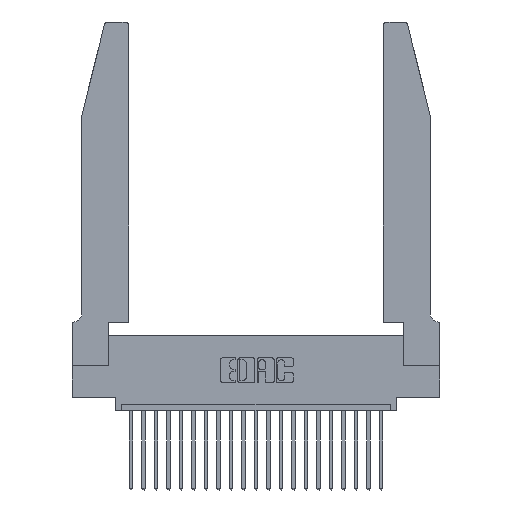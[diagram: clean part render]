
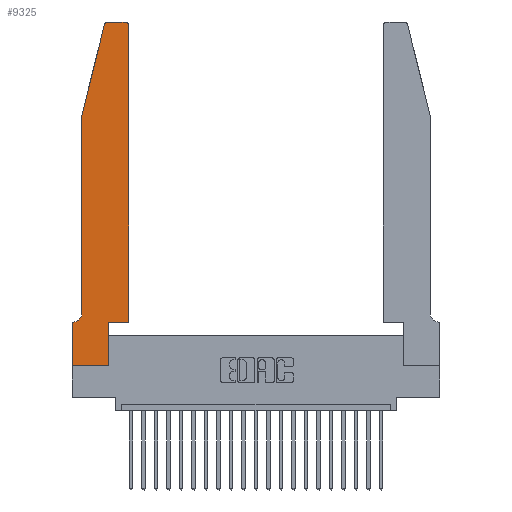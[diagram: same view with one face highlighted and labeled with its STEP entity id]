
A CAD part, top view. The second image highlights one B-rep face of the part: STEP entity #9325.
In plain terms, the highlighted planar face has unit normal (0, 0, 1).
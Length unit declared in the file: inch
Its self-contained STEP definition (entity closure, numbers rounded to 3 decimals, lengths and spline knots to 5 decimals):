
#267 = CARTESIAN_POINT ( 'NONE',  ( 0.0755, 2., 0.37 ) ) ;
#661 = VECTOR ( 'NONE', #10644, 39.37008 ) ;
#750 = VECTOR ( 'NONE', #2296, 39.37008 ) ;
#885 = ORIENTED_EDGE ( 'NONE', *, *, #1865, .T. ) ;
#1027 = CARTESIAN_POINT ( 'NONE',  ( 0.0755, 2., 0.37 ) ) ;
#1036 = CARTESIAN_POINT ( 'NONE',  ( 0., 0., 0.37 ) ) ;
#1344 = LINE ( 'NONE', #19216, #16714 ) ;
#1485 = FACE_OUTER_BOUND ( 'NONE', #23130, .T. ) ;
#1508 = CARTESIAN_POINT ( 'NONE',  ( 0.0055, 0.35, 0.37 ) ) ;
#1568 = EDGE_CURVE ( 'NONE', #22589, #5425, #1344, .T. ) ;
#1865 = EDGE_CURVE ( 'NONE', #16413, #19247, #22656, .T. ) ;
#2060 = ORIENTED_EDGE ( 'NONE', *, *, #14155, .T. ) ;
#2296 = DIRECTION ( 'NONE',  ( -1., 0., 0. ) ) ;
#2621 = AXIS2_PLACEMENT_3D ( 'NONE', #10763, #23395, #11140 ) ;
#2838 = DIRECTION ( 'NONE',  ( 1., 0., 0. ) ) ;
#2913 = EDGE_CURVE ( 'NONE', #19247, #7035, #15237, .T. ) ;
#2962 = CARTESIAN_POINT ( 'NONE',  ( 0.2865, 0., 0.37 ) ) ;
#3197 = AXIS2_PLACEMENT_3D ( 'NONE', #18968, #13640, #6188 ) ;
#3461 = AXIS2_PLACEMENT_3D ( 'NONE', #21875, #18325, #22052 ) ;
#3768 = ORIENTED_EDGE ( 'NONE', *, *, #13486, .T. ) ;
#3876 = EDGE_CURVE ( 'NONE', #15481, #22604, #21667, .T. ) ;
#3895 = CARTESIAN_POINT ( 'NONE',  ( 0.0755, 2., 0.37 ) ) ;
#5021 = EDGE_CURVE ( 'NONE', #11705, #9742, #11743, .T. ) ;
#5425 = VERTEX_POINT ( 'NONE', #19718 ) ;
#5506 = LINE ( 'NONE', #6840, #661 ) ;
#5537 = PLANE ( 'NONE',  #3461 ) ;
#6188 = DIRECTION ( 'NONE',  ( -1., 0., 0. ) ) ;
#6190 = CARTESIAN_POINT ( 'NONE',  ( 0.284, 2.75, 0.37 ) ) ;
#6840 = CARTESIAN_POINT ( 'NONE',  ( 0.4505, 0.35, 0.37 ) ) ;
#7035 = VERTEX_POINT ( 'NONE', #21923 ) ;
#7165 = ORIENTED_EDGE ( 'NONE', *, *, #3876, .T. ) ;
#7167 = VECTOR ( 'NONE', #9153, 39.37008 ) ;
#7183 = VERTEX_POINT ( 'NONE', #2962 ) ;
#7184 = VECTOR ( 'NONE', #10777, 39.37008 ) ;
#7331 = DIRECTION ( 'NONE',  ( 0., 0., 1. ) ) ;
#7676 = ORIENTED_EDGE ( 'NONE', *, *, #2913, .T. ) ;
#7879 = CARTESIAN_POINT ( 'NONE',  ( 0.4505, 2.72, 0.37 ) ) ;
#8129 = ORIENTED_EDGE ( 'NONE', *, *, #15659, .T. ) ;
#8847 = DIRECTION ( 'NONE',  ( -1., 0., 0. ) ) ;
#8895 = EDGE_CURVE ( 'NONE', #22604, #11705, #16934, .T. ) ;
#9153 = DIRECTION ( 'NONE',  ( 0., -1., 0. ) ) ;
#9206 = ORIENTED_EDGE ( 'NONE', *, *, #5021, .T. ) ;
#9325 = ADVANCED_FACE ( 'NONE', ( #1485 ), #5537, .T. ) ;
#9742 = VERTEX_POINT ( 'NONE', #3895 ) ;
#10244 = ORIENTED_EDGE ( 'NONE', *, *, #15601, .T. ) ;
#10644 = DIRECTION ( 'NONE',  ( 0., 1., 0. ) ) ;
#10763 = CARTESIAN_POINT ( 'NONE',  ( 0.4205, 2.72, 0.37 ) ) ;
#10777 = DIRECTION ( 'NONE',  ( 0., 1., 0. ) ) ;
#10817 = EDGE_CURVE ( 'NONE', #11311, #16413, #23236, .T. ) ;
#11140 = DIRECTION ( 'NONE',  ( 1., 0., 0. ) ) ;
#11311 = VERTEX_POINT ( 'NONE', #21190 ) ;
#11705 = VERTEX_POINT ( 'NONE', #22453 ) ;
#11743 = LINE ( 'NONE', #1027, #14251 ) ;
#12129 = DIRECTION ( 'NONE',  ( 0., -1., 0. ) ) ;
#12845 = VECTOR ( 'NONE', #8847, 39.37008 ) ;
#13413 = ORIENTED_EDGE ( 'NONE', *, *, #8895, .T. ) ;
#13444 = ORIENTED_EDGE ( 'NONE', *, *, #1568, .T. ) ;
#13486 = EDGE_CURVE ( 'NONE', #5425, #19635, #5506, .T. ) ;
#13640 = DIRECTION ( 'NONE',  ( 0., 0., -1. ) ) ;
#13736 = LINE ( 'NONE', #15123, #14837 ) ;
#14155 = EDGE_CURVE ( 'NONE', #7035, #7183, #13736, .T. ) ;
#14251 = VECTOR ( 'NONE', #17419, 39.37008 ) ;
#14837 = VECTOR ( 'NONE', #18871, 39.37008 ) ;
#15123 = CARTESIAN_POINT ( 'NONE',  ( 0., 0., 0.37 ) ) ;
#15237 = LINE ( 'NONE', #1036, #19240 ) ;
#15369 = CARTESIAN_POINT ( 'NONE',  ( 0.4205, 2.75, 0.37 ) ) ;
#15481 = VERTEX_POINT ( 'NONE', #15369 ) ;
#15601 = EDGE_CURVE ( 'NONE', #19635, #15481, #21363, .T. ) ;
#15659 = EDGE_CURVE ( 'NONE', #9742, #11311, #15972, .T. ) ;
#15972 = LINE ( 'NONE', #267, #7167 ) ;
#16413 = VERTEX_POINT ( 'NONE', #1508 ) ;
#16556 = LINE ( 'NONE', #21605, #7184 ) ;
#16714 = VECTOR ( 'NONE', #2838, 39.37008 ) ;
#16934 = CIRCLE ( 'NONE', #17028, 0.03 ) ;
#17028 = AXIS2_PLACEMENT_3D ( 'NONE', #18056, #7331, #18127 ) ;
#17295 = ORIENTED_EDGE ( 'NONE', *, *, #10817, .T. ) ;
#17419 = DIRECTION ( 'NONE',  ( -0.239, -0.971, 0. ) ) ;
#18056 = CARTESIAN_POINT ( 'NONE',  ( 0.284, 2.72, 0.37 ) ) ;
#18127 = DIRECTION ( 'NONE',  ( 1., 0., 0. ) ) ;
#18325 = DIRECTION ( 'NONE',  ( 0., 0., 1. ) ) ;
#18871 = DIRECTION ( 'NONE',  ( 1., 0., 0. ) ) ;
#18968 = CARTESIAN_POINT ( 'NONE',  ( 0.0055, 0.42, 0.37 ) ) ;
#19216 = CARTESIAN_POINT ( 'NONE',  ( 0.4505, 0.35, 0.37 ) ) ;
#19240 = VECTOR ( 'NONE', #12129, 39.37008 ) ;
#19247 = VERTEX_POINT ( 'NONE', #20449 ) ;
#19264 = CARTESIAN_POINT ( 'NONE',  ( 0.2605, 2.75, 0.37 ) ) ;
#19635 = VERTEX_POINT ( 'NONE', #7879 ) ;
#19718 = CARTESIAN_POINT ( 'NONE',  ( 0.4505, 0.35, 0.37 ) ) ;
#20449 = CARTESIAN_POINT ( 'NONE',  ( 0., 0.35, 0.37 ) ) ;
#20574 = EDGE_CURVE ( 'NONE', #7183, #22589, #16556, .T. ) ;
#20664 = ORIENTED_EDGE ( 'NONE', *, *, #20574, .T. ) ;
#21190 = CARTESIAN_POINT ( 'NONE',  ( 0.0755, 0.42, 0.37 ) ) ;
#21363 = CIRCLE ( 'NONE', #2621, 0.03 ) ;
#21605 = CARTESIAN_POINT ( 'NONE',  ( 0.2865, 0.35, 0.37 ) ) ;
#21667 = LINE ( 'NONE', #19264, #12845 ) ;
#21875 = CARTESIAN_POINT ( 'NONE',  ( 0., 0.35, 0.37 ) ) ;
#21923 = CARTESIAN_POINT ( 'NONE',  ( 0., 0., 0.37 ) ) ;
#21988 = CARTESIAN_POINT ( 'NONE',  ( 0.0755, 0.35, 0.37 ) ) ;
#22052 = DIRECTION ( 'NONE',  ( 1., 0., 0. ) ) ;
#22453 = CARTESIAN_POINT ( 'NONE',  ( 0.25487, 2.72718, 0.37 ) ) ;
#22589 = VERTEX_POINT ( 'NONE', #22997 ) ;
#22604 = VERTEX_POINT ( 'NONE', #6190 ) ;
#22656 = LINE ( 'NONE', #21988, #750 ) ;
#22997 = CARTESIAN_POINT ( 'NONE',  ( 0.2865, 0.35, 0.37 ) ) ;
#23130 = EDGE_LOOP ( 'NONE', ( #7165, #13413, #9206, #8129, #17295, #885, #7676, #2060, #20664, #13444, #3768, #10244 ) ) ;
#23236 = CIRCLE ( 'NONE', #3197, 0.07 ) ;
#23395 = DIRECTION ( 'NONE',  ( 0., 0., 1. ) ) ;
